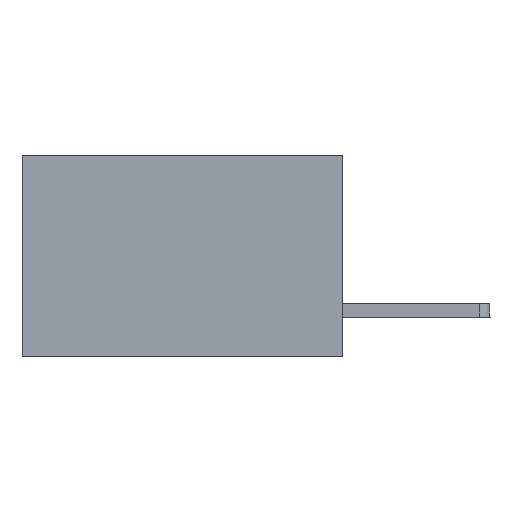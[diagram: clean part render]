
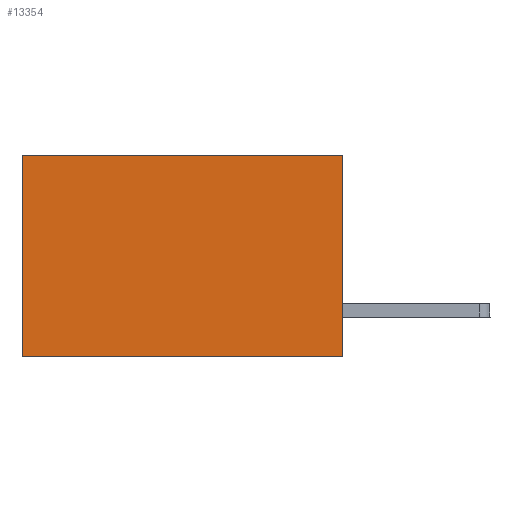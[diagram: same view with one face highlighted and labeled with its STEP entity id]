
A CAD part, left-side view. The second image highlights one B-rep face of the part: STEP entity #13354.
In plain terms, the highlighted planar face has unit normal (-1, 0, 0).
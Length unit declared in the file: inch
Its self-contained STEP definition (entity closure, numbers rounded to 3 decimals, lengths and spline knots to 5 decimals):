
#85 = ORIENTED_EDGE ( 'NONE', *, *, #7779, .T. ) ;
#98 = CARTESIAN_POINT ( 'NONE',  ( 0.277, 0.59, 0. ) ) ;
#106 = ORIENTED_EDGE ( 'NONE', *, *, #229, .F. ) ;
#229 = EDGE_CURVE ( 'NONE', #12958, #8502, #8414, .T. ) ;
#390 = CARTESIAN_POINT ( 'NONE',  ( 0.277, 0., 0. ) ) ;
#558 = CARTESIAN_POINT ( 'NONE',  ( 0.277, 0., 0. ) ) ;
#1270 = CARTESIAN_POINT ( 'NONE',  ( 0.277, 0.59, -0.37 ) ) ;
#2327 = VERTEX_POINT ( 'NONE', #98 ) ;
#3390 = DIRECTION ( 'NONE',  ( 0., 0., -1. ) ) ;
#3652 = EDGE_CURVE ( 'NONE', #6081, #2327, #6271, .T. ) ;
#3759 = EDGE_CURVE ( 'NONE', #6081, #12958, #5412, .T. ) ;
#4354 = PLANE ( 'NONE',  #5332 ) ;
#4770 = VECTOR ( 'NONE', #10811, 39.37008 ) ;
#5332 = AXIS2_PLACEMENT_3D ( 'NONE', #13451, #11016, #3390 ) ;
#5354 = ORIENTED_EDGE ( 'NONE', *, *, #3652, .T. ) ;
#5412 = LINE ( 'NONE', #13011, #4770 ) ;
#5465 = ORIENTED_EDGE ( 'NONE', *, *, #3759, .F. ) ;
#6081 = VERTEX_POINT ( 'NONE', #390 ) ;
#6271 = LINE ( 'NONE', #558, #10015 ) ;
#6580 = FACE_OUTER_BOUND ( 'NONE', #12196, .T. ) ;
#7171 = VECTOR ( 'NONE', #10412, 39.37008 ) ;
#7518 = LINE ( 'NONE', #13123, #8357 ) ;
#7779 = EDGE_CURVE ( 'NONE', #2327, #8502, #7518, .T. ) ;
#8357 = VECTOR ( 'NONE', #11133, 39.37008 ) ;
#8414 = LINE ( 'NONE', #12900, #7171 ) ;
#8502 = VERTEX_POINT ( 'NONE', #1270 ) ;
#8711 = DIRECTION ( 'NONE',  ( 0., 1., 0. ) ) ;
#10015 = VECTOR ( 'NONE', #8711, 39.37008 ) ;
#10412 = DIRECTION ( 'NONE',  ( 0., 1., 0. ) ) ;
#10811 = DIRECTION ( 'NONE',  ( 0., 0., -1. ) ) ;
#11016 = DIRECTION ( 'NONE',  ( 1., 0., 0. ) ) ;
#11133 = DIRECTION ( 'NONE',  ( 0., 0., -1. ) ) ;
#12196 = EDGE_LOOP ( 'NONE', ( #85, #106, #5465, #5354 ) ) ;
#12900 = CARTESIAN_POINT ( 'NONE',  ( 0.277, 0., -0.37 ) ) ;
#12958 = VERTEX_POINT ( 'NONE', #14358 ) ;
#13011 = CARTESIAN_POINT ( 'NONE',  ( 0.277, 0., -0.37 ) ) ;
#13123 = CARTESIAN_POINT ( 'NONE',  ( 0.277, 0.59, -0.37 ) ) ;
#13354 = ADVANCED_FACE ( 'NONE', ( #6580 ), #4354, .F. ) ;
#13451 = CARTESIAN_POINT ( 'NONE',  ( 0.277, 0., -0.37 ) ) ;
#14358 = CARTESIAN_POINT ( 'NONE',  ( 0.277, 0., -0.37 ) ) ;
